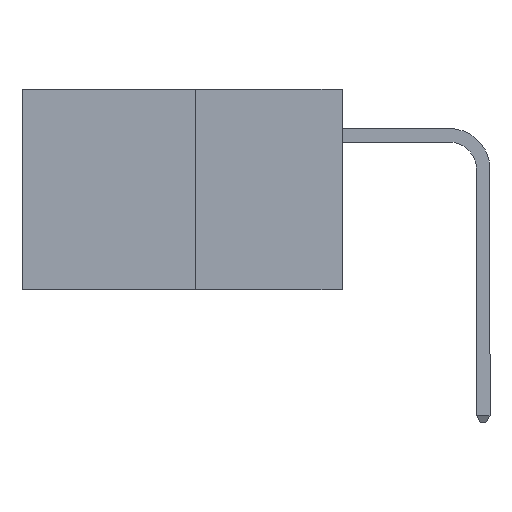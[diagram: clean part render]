
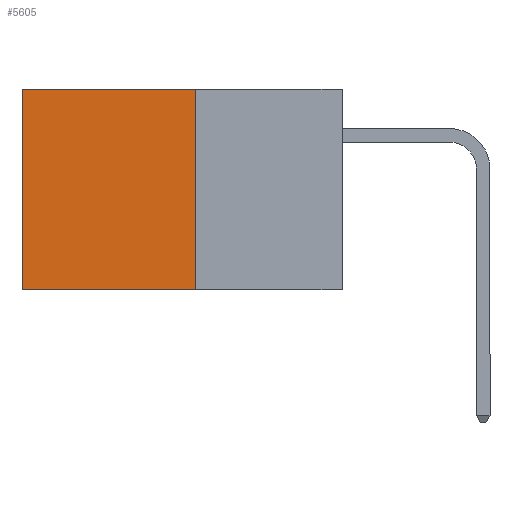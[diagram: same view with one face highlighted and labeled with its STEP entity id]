
A CAD part, left-side view. The second image highlights one B-rep face of the part: STEP entity #5605.
In plain terms, the highlighted planar face has unit normal (-1, 0, 0).
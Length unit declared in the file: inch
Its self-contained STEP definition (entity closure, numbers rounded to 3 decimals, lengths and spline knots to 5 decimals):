
#216 = DIRECTION ( 'NONE',  ( 0., 0., -1. ) ) ;
#250 = CARTESIAN_POINT ( 'NONE',  ( 0.277, 0.27, -0.37 ) ) ;
#344 = ORIENTED_EDGE ( 'NONE', *, *, #7562, .F. ) ;
#437 = VERTEX_POINT ( 'NONE', #2834 ) ;
#622 = DIRECTION ( 'NONE',  ( 0., 0., -1. ) ) ;
#632 = PLANE ( 'NONE',  #5416 ) ;
#659 = DIRECTION ( 'NONE',  ( 1., 0., 0. ) ) ;
#761 = CARTESIAN_POINT ( 'NONE',  ( 0.277, 0.27, -0.37 ) ) ;
#793 = LINE ( 'NONE', #6960, #8029 ) ;
#873 = CARTESIAN_POINT ( 'NONE',  ( 0.277, 0.27, -0.37 ) ) ;
#963 = FACE_OUTER_BOUND ( 'NONE', #2573, .T. ) ;
#1593 = ORIENTED_EDGE ( 'NONE', *, *, #8878, .T. ) ;
#1770 = ORIENTED_EDGE ( 'NONE', *, *, #1938, .T. ) ;
#1938 = EDGE_CURVE ( 'NONE', #6072, #437, #2213, .T. ) ;
#2213 = LINE ( 'NONE', #7405, #9116 ) ;
#2395 = LINE ( 'NONE', #250, #4049 ) ;
#2453 = VERTEX_POINT ( 'NONE', #7101 ) ;
#2573 = EDGE_LOOP ( 'NONE', ( #1593, #2657, #344, #1770 ) ) ;
#2657 = ORIENTED_EDGE ( 'NONE', *, *, #5878, .F. ) ;
#2834 = CARTESIAN_POINT ( 'NONE',  ( 0.277, 0.59, 0. ) ) ;
#3520 = VECTOR ( 'NONE', #8187, 39.37008 ) ;
#4049 = VECTOR ( 'NONE', #216, 39.37008 ) ;
#5416 = AXIS2_PLACEMENT_3D ( 'NONE', #761, #659, #622 ) ;
#5605 = ADVANCED_FACE ( 'NONE', ( #963 ), #632, .F. ) ;
#5825 = LINE ( 'NONE', #8100, #3520 ) ;
#5878 = EDGE_CURVE ( 'NONE', #6279, #2453, #5825, .T. ) ;
#6072 = VERTEX_POINT ( 'NONE', #7198 ) ;
#6279 = VERTEX_POINT ( 'NONE', #873 ) ;
#6960 = CARTESIAN_POINT ( 'NONE',  ( 0.277, 0.59, -0.37 ) ) ;
#6988 = DIRECTION ( 'NONE',  ( 0., 0., -1. ) ) ;
#7101 = CARTESIAN_POINT ( 'NONE',  ( 0.277, 0.59, -0.37 ) ) ;
#7198 = CARTESIAN_POINT ( 'NONE',  ( 0.277, 0.27, 0. ) ) ;
#7405 = CARTESIAN_POINT ( 'NONE',  ( 0.277, 0.27, 0. ) ) ;
#7562 = EDGE_CURVE ( 'NONE', #6072, #6279, #2395, .T. ) ;
#8029 = VECTOR ( 'NONE', #6988, 39.37008 ) ;
#8100 = CARTESIAN_POINT ( 'NONE',  ( 0.277, 0.27, -0.37 ) ) ;
#8187 = DIRECTION ( 'NONE',  ( 0., 1., 0. ) ) ;
#8878 = EDGE_CURVE ( 'NONE', #437, #2453, #793, .T. ) ;
#8907 = DIRECTION ( 'NONE',  ( 0., 1., 0. ) ) ;
#9116 = VECTOR ( 'NONE', #8907, 39.37008 ) ;
